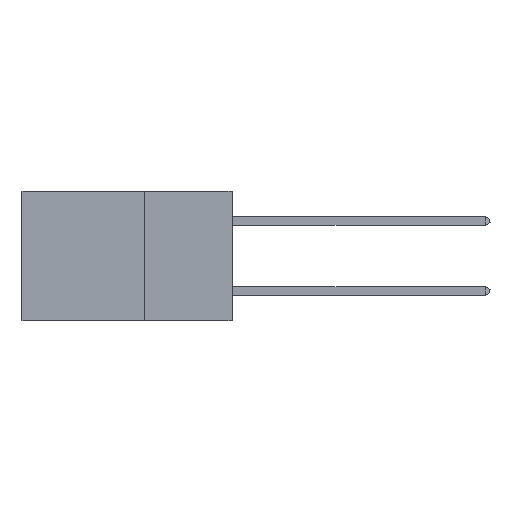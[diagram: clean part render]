
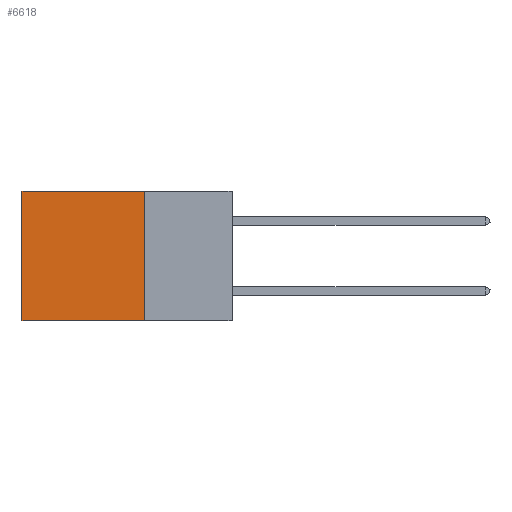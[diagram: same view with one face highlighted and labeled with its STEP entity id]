
A CAD part, left-side view. The second image highlights one B-rep face of the part: STEP entity #6618.
In plain terms, the highlighted planar face has unit normal (-1, 0, 0).
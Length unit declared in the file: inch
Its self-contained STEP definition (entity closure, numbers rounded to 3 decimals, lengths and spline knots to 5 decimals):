
#395 = LINE ( 'NONE', #14372, #9526 ) ;
#613 = CARTESIAN_POINT ( 'NONE',  ( 0.2875, 0.6, -0.37 ) ) ;
#1049 = VECTOR ( 'NONE', #15180, 39.37008 ) ;
#1796 = VERTEX_POINT ( 'NONE', #2851 ) ;
#2728 = ORIENTED_EDGE ( 'NONE', *, *, #14826, .F. ) ;
#2851 = CARTESIAN_POINT ( 'NONE',  ( 0.2875, 0.25, 0. ) ) ;
#3278 = LINE ( 'NONE', #4764, #7238 ) ;
#3645 = CARTESIAN_POINT ( 'NONE',  ( 0.2875, 0.25, -0.37 ) ) ;
#3830 = EDGE_CURVE ( 'NONE', #1796, #4014, #5624, .T. ) ;
#4014 = VERTEX_POINT ( 'NONE', #18867 ) ;
#4203 = FACE_OUTER_BOUND ( 'NONE', #17864, .T. ) ;
#4764 = CARTESIAN_POINT ( 'NONE',  ( 0.2875, 0.25, 0. ) ) ;
#5624 = LINE ( 'NONE', #16028, #1049 ) ;
#6618 = ADVANCED_FACE ( 'NONE', ( #4203 ), #10595, .F. ) ;
#6817 = EDGE_CURVE ( 'NONE', #4014, #17444, #395, .T. ) ;
#7238 = VECTOR ( 'NONE', #8190, 39.37008 ) ;
#7822 = VECTOR ( 'NONE', #16962, 39.37008 ) ;
#8190 = DIRECTION ( 'NONE',  ( 0., 0., -1. ) ) ;
#8497 = AXIS2_PLACEMENT_3D ( 'NONE', #18848, #9021, #20492 ) ;
#9021 = DIRECTION ( 'NONE',  ( 1., 0., 0. ) ) ;
#9389 = ORIENTED_EDGE ( 'NONE', *, *, #6817, .T. ) ;
#9465 = DIRECTION ( 'NONE',  ( 0., 0., -1. ) ) ;
#9526 = VECTOR ( 'NONE', #9465, 39.37008 ) ;
#9763 = VERTEX_POINT ( 'NONE', #14595 ) ;
#10595 = PLANE ( 'NONE',  #8497 ) ;
#11255 = EDGE_CURVE ( 'NONE', #9763, #17444, #20926, .T. ) ;
#14372 = CARTESIAN_POINT ( 'NONE',  ( 0.2875, 0.6, 0. ) ) ;
#14595 = CARTESIAN_POINT ( 'NONE',  ( 0.2875, 0.25, -0.37 ) ) ;
#14826 = EDGE_CURVE ( 'NONE', #1796, #9763, #3278, .T. ) ;
#15180 = DIRECTION ( 'NONE',  ( 0., 1., 0. ) ) ;
#16028 = CARTESIAN_POINT ( 'NONE',  ( 0.2875, 0.25, 0. ) ) ;
#16962 = DIRECTION ( 'NONE',  ( 0., 1., 0. ) ) ;
#17421 = ORIENTED_EDGE ( 'NONE', *, *, #3830, .T. ) ;
#17444 = VERTEX_POINT ( 'NONE', #613 ) ;
#17864 = EDGE_LOOP ( 'NONE', ( #9389, #18703, #2728, #17421 ) ) ;
#18703 = ORIENTED_EDGE ( 'NONE', *, *, #11255, .F. ) ;
#18848 = CARTESIAN_POINT ( 'NONE',  ( 0.2875, 0.25, 0. ) ) ;
#18867 = CARTESIAN_POINT ( 'NONE',  ( 0.2875, 0.6, 0. ) ) ;
#20492 = DIRECTION ( 'NONE',  ( 0., 0., -1. ) ) ;
#20926 = LINE ( 'NONE', #3645, #7822 ) ;
